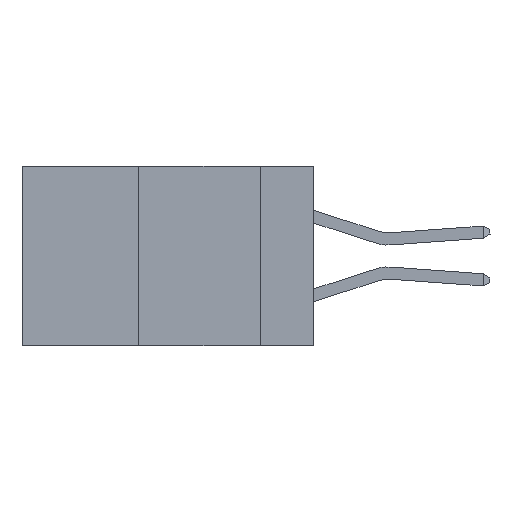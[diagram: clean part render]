
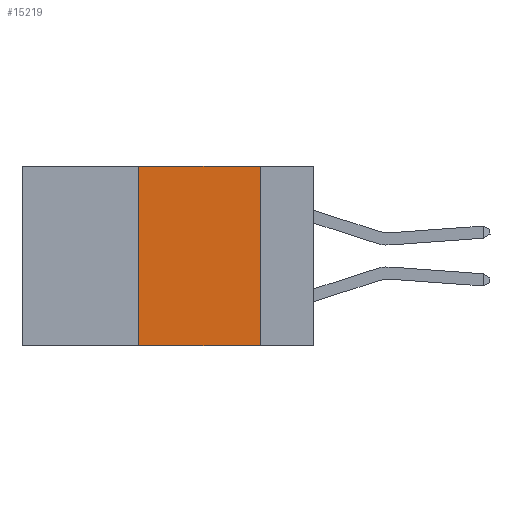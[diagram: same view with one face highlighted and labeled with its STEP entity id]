
A CAD part, left-side view. The second image highlights one B-rep face of the part: STEP entity #15219.
In plain terms, the highlighted planar face has unit normal (-1, 0, 0).
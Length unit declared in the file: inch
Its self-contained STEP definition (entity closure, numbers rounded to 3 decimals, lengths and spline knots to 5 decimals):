
#745 = ORIENTED_EDGE ( 'NONE', *, *, #23618, .T. ) ;
#853 = EDGE_CURVE ( 'NONE', #1700, #19066, #3619, .T. ) ;
#1700 = VERTEX_POINT ( 'NONE', #4443 ) ;
#3159 = CARTESIAN_POINT ( 'NONE',  ( 0., 0.6, 0. ) ) ;
#3619 = LINE ( 'NONE', #6605, #21818 ) ;
#4221 = CARTESIAN_POINT ( 'NONE',  ( 0., 0.36, 0. ) ) ;
#4443 = CARTESIAN_POINT ( 'NONE',  ( 0., 0.36, 0. ) ) ;
#6605 = CARTESIAN_POINT ( 'NONE',  ( 0., 0.6, 0. ) ) ;
#10134 = PLANE ( 'NONE',  #26959 ) ;
#11702 = CARTESIAN_POINT ( 'NONE',  ( 0., 0.11, -0.37 ) ) ;
#12822 = EDGE_LOOP ( 'NONE', ( #13998, #32517, #22273, #745 ) ) ;
#13998 = ORIENTED_EDGE ( 'NONE', *, *, #16173, .F. ) ;
#15219 = ADVANCED_FACE ( 'NONE', ( #25119 ), #10134, .F. ) ;
#15327 = DIRECTION ( 'NONE',  ( 1., 0., 0. ) ) ;
#15806 = LINE ( 'NONE', #4221, #21896 ) ;
#16173 = EDGE_CURVE ( 'NONE', #19066, #26887, #37439, .T. ) ;
#16893 = LINE ( 'NONE', #23062, #24022 ) ;
#19066 = VERTEX_POINT ( 'NONE', #22818 ) ;
#19543 = EDGE_CURVE ( 'NONE', #24431, #1700, #15806, .T. ) ;
#19797 = CARTESIAN_POINT ( 'NONE',  ( 0., 0.11, 0. ) ) ;
#21818 = VECTOR ( 'NONE', #30986, 39.37008 ) ;
#21896 = VECTOR ( 'NONE', #21993, 39.37008 ) ;
#21993 = DIRECTION ( 'NONE',  ( 0., 0., 1. ) ) ;
#22273 = ORIENTED_EDGE ( 'NONE', *, *, #19543, .F. ) ;
#22818 = CARTESIAN_POINT ( 'NONE',  ( 0., 0.11, 0. ) ) ;
#23062 = CARTESIAN_POINT ( 'NONE',  ( 0., 0.6, -0.37 ) ) ;
#23618 = EDGE_CURVE ( 'NONE', #24431, #26887, #16893, .T. ) ;
#24022 = VECTOR ( 'NONE', #29287, 39.37008 ) ;
#24431 = VERTEX_POINT ( 'NONE', #32402 ) ;
#25119 = FACE_OUTER_BOUND ( 'NONE', #12822, .T. ) ;
#25728 = VECTOR ( 'NONE', #35196, 39.37008 ) ;
#26887 = VERTEX_POINT ( 'NONE', #11702 ) ;
#26959 = AXIS2_PLACEMENT_3D ( 'NONE', #3159, #15327, #33727 ) ;
#29287 = DIRECTION ( 'NONE',  ( 0., -1., 0. ) ) ;
#30986 = DIRECTION ( 'NONE',  ( 0., -1., 0. ) ) ;
#32402 = CARTESIAN_POINT ( 'NONE',  ( 0., 0.36, -0.37 ) ) ;
#32517 = ORIENTED_EDGE ( 'NONE', *, *, #853, .F. ) ;
#33727 = DIRECTION ( 'NONE',  ( 0., 0., -1. ) ) ;
#35196 = DIRECTION ( 'NONE',  ( 0., 0., -1. ) ) ;
#37439 = LINE ( 'NONE', #19797, #25728 ) ;
